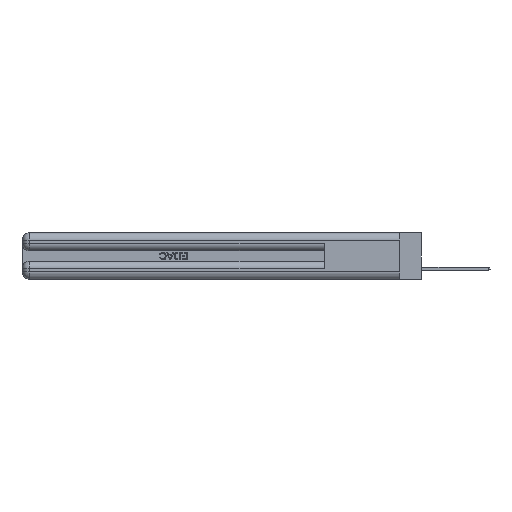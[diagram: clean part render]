
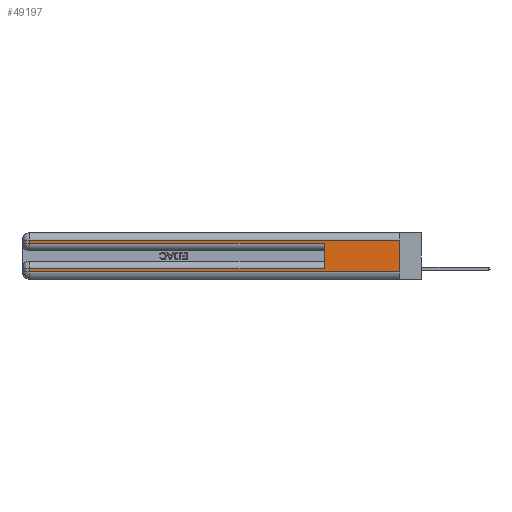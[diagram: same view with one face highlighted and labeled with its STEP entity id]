
A CAD part, left-side view. The second image highlights one B-rep face of the part: STEP entity #49197.
In plain terms, the highlighted planar face has unit normal (-1, 0, 0).
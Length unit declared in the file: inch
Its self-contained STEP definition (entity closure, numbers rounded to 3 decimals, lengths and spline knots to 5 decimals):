
#244 = DIRECTION ( 'NONE',  ( 0., 1., 0. ) ) ;
#419 = EDGE_CURVE ( 'NONE', #46622, #42552, #3919, .T. ) ;
#660 = CARTESIAN_POINT ( 'NONE',  ( 0., 2.94, 0.285 ) ) ;
#662 = EDGE_CURVE ( 'NONE', #40881, #36366, #23773, .T. ) ;
#1923 = VECTOR ( 'NONE', #35974, 39.37008 ) ;
#2125 = PLANE ( 'NONE',  #46002 ) ;
#2209 = DIRECTION ( 'NONE',  ( 0., 0., -1. ) ) ;
#2515 = ORIENTED_EDGE ( 'NONE', *, *, #15336, .F. ) ;
#2599 = CARTESIAN_POINT ( 'NONE',  ( 0., 2.94, 0.31 ) ) ;
#2806 = CARTESIAN_POINT ( 'NONE',  ( 0., 2.94, 0.37 ) ) ;
#2848 = EDGE_CURVE ( 'NONE', #36366, #24484, #24274, .T. ) ;
#3005 = DIRECTION ( 'NONE',  ( 0., 0., 1. ) ) ;
#3919 = LINE ( 'NONE', #2806, #38330 ) ;
#5140 = LINE ( 'NONE', #40418, #22136 ) ;
#5499 = CARTESIAN_POINT ( 'NONE',  ( 0., 0.6, 0.285 ) ) ;
#7292 = EDGE_CURVE ( 'NONE', #42552, #22149, #5140, .T. ) ;
#7359 = CARTESIAN_POINT ( 'NONE',  ( 0., 0., 0.37 ) ) ;
#8890 = LINE ( 'NONE', #40118, #13789 ) ;
#9616 = CARTESIAN_POINT ( 'NONE',  ( 0., 0., 0.085 ) ) ;
#9937 = VECTOR ( 'NONE', #3005, 39.37008 ) ;
#10916 = CARTESIAN_POINT ( 'NONE',  ( 0., 2.94, 0.06 ) ) ;
#12081 = CARTESIAN_POINT ( 'NONE',  ( 0., 0.6, 0.085 ) ) ;
#12430 = EDGE_CURVE ( 'NONE', #25398, #40881, #35086, .T. ) ;
#12852 = ORIENTED_EDGE ( 'NONE', *, *, #40086, .F. ) ;
#13789 = VECTOR ( 'NONE', #2209, 39.37008 ) ;
#15336 = EDGE_CURVE ( 'NONE', #25398, #22149, #26936, .T. ) ;
#15342 = VECTOR ( 'NONE', #39551, 39.37008 ) ;
#16874 = ORIENTED_EDGE ( 'NONE', *, *, #7292, .T. ) ;
#17987 = VERTEX_POINT ( 'NONE', #45419 ) ;
#18490 = DIRECTION ( 'NONE',  ( 0., 0., -1. ) ) ;
#18820 = DIRECTION ( 'NONE',  ( 1., 0., 0. ) ) ;
#20884 = ORIENTED_EDGE ( 'NONE', *, *, #419, .T. ) ;
#21052 = DIRECTION ( 'NONE',  ( 0., -1., 0. ) ) ;
#21208 = CARTESIAN_POINT ( 'NONE',  ( 0., 0., 0.06 ) ) ;
#22136 = VECTOR ( 'NONE', #21052, 39.37008 ) ;
#22149 = VERTEX_POINT ( 'NONE', #5499 ) ;
#23773 = LINE ( 'NONE', #39714, #15342 ) ;
#24274 = LINE ( 'NONE', #48288, #1923 ) ;
#24484 = VERTEX_POINT ( 'NONE', #21208 ) ;
#25060 = EDGE_LOOP ( 'NONE', ( #12852, #29404, #20884, #16874, #2515, #47006, #47347, #48885 ) ) ;
#25398 = VERTEX_POINT ( 'NONE', #12081 ) ;
#26936 = LINE ( 'NONE', #41973, #9937 ) ;
#27819 = VECTOR ( 'NONE', #40178, 39.37008 ) ;
#28745 = FACE_OUTER_BOUND ( 'NONE', #25060, .T. ) ;
#29404 = ORIENTED_EDGE ( 'NONE', *, *, #42440, .T. ) ;
#31080 = VECTOR ( 'NONE', #244, 39.37008 ) ;
#34381 = DIRECTION ( 'NONE',  ( 0., 0., -1. ) ) ;
#35086 = LINE ( 'NONE', #9616, #27819 ) ;
#35974 = DIRECTION ( 'NONE',  ( 0., -1., 0. ) ) ;
#36366 = VERTEX_POINT ( 'NONE', #10916 ) ;
#38330 = VECTOR ( 'NONE', #18490, 39.37008 ) ;
#39551 = DIRECTION ( 'NONE',  ( 0., 0., -1. ) ) ;
#39714 = CARTESIAN_POINT ( 'NONE',  ( 0., 2.94, 0.37 ) ) ;
#40086 = EDGE_CURVE ( 'NONE', #17987, #24484, #8890, .T. ) ;
#40118 = CARTESIAN_POINT ( 'NONE',  ( 0., 0., 0.37 ) ) ;
#40178 = DIRECTION ( 'NONE',  ( 0., 1., 0. ) ) ;
#40418 = CARTESIAN_POINT ( 'NONE',  ( 0., 0., 0.285 ) ) ;
#40881 = VERTEX_POINT ( 'NONE', #45663 ) ;
#41973 = CARTESIAN_POINT ( 'NONE',  ( 0., 0.6, 0.145 ) ) ;
#42440 = EDGE_CURVE ( 'NONE', #17987, #46622, #44317, .T. ) ;
#42552 = VERTEX_POINT ( 'NONE', #660 ) ;
#44317 = LINE ( 'NONE', #46274, #31080 ) ;
#45419 = CARTESIAN_POINT ( 'NONE',  ( 0., 0., 0.31 ) ) ;
#45663 = CARTESIAN_POINT ( 'NONE',  ( 0., 2.94, 0.085 ) ) ;
#46002 = AXIS2_PLACEMENT_3D ( 'NONE', #7359, #18820, #34381 ) ;
#46274 = CARTESIAN_POINT ( 'NONE',  ( 0., 0., 0.31 ) ) ;
#46622 = VERTEX_POINT ( 'NONE', #2599 ) ;
#47006 = ORIENTED_EDGE ( 'NONE', *, *, #12430, .T. ) ;
#47347 = ORIENTED_EDGE ( 'NONE', *, *, #662, .T. ) ;
#48288 = CARTESIAN_POINT ( 'NONE',  ( 0., 0., 0.06 ) ) ;
#48885 = ORIENTED_EDGE ( 'NONE', *, *, #2848, .T. ) ;
#49197 = ADVANCED_FACE ( 'NONE', ( #28745 ), #2125, .F. ) ;
